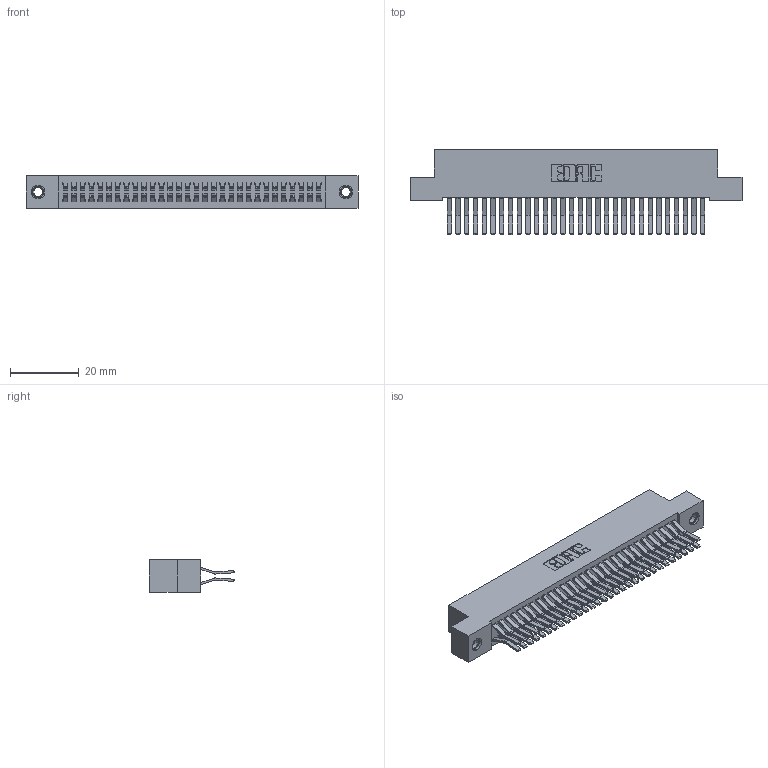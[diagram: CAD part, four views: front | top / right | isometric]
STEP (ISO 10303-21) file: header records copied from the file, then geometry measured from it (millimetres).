
FILE_DESCRIPTION (( 'STEP AP203' ), '1' );
FILE_NAME ('342-060-560-207.STEP', '2018-08-13T06:28:00', ( '' ), ( '' ), 'SwSTEP 2.0', 'SolidWorks 2016', '' );
FILE_SCHEMA (( 'CONFIG_CONTROL_DESIGN' ));
Length unit declared in the file: inch
Products named in the file (4): 342 Part_TI; 345-292-001_560 Tail; 345-250-001_345-250-005-103; 342-060-560-207
Assembly tree (63 placements, depth 2):
  342-060-560-207
    342 Part_TI
    345-292-001_560 Tail  x60
    345-250-001_345-250-005-103  x2
Bounding box: 96.52 x 24.78 x 9.4 mm (x, y, z)
Volume: 8996.7 mm3; surface area: 15319.1 mm2
Topology: 63 solids, 63 shells, 3410 faces, 10095 edges, 6642 vertices
Faces by surface type: plane 2258, cylinder 1136, cone 12, torus 4
Entity records: 21994 total; most frequent: CARTESIAN_POINT 3641, ORIENTED_EDGE 3570, DIRECTION 3167, EDGE_CURVE 1785, VECTOR 1633, LINE 1633, VERTEX_POINT 1184, AXIS2_PLACEMENT_3D 767
